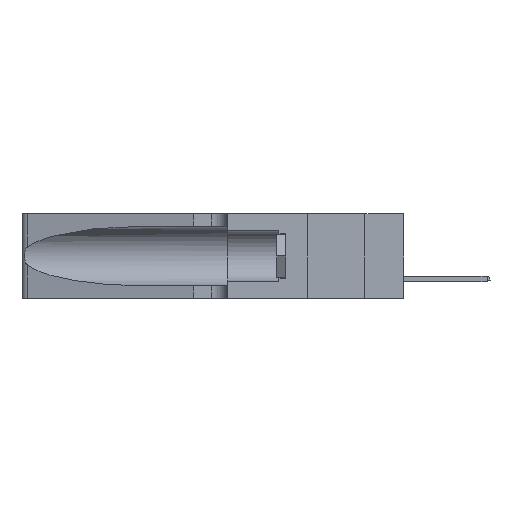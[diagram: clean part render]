
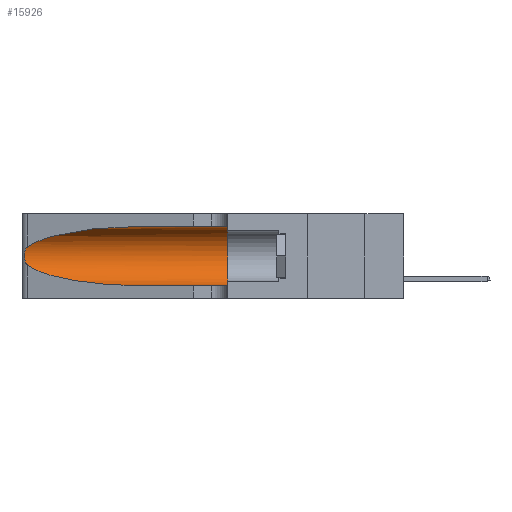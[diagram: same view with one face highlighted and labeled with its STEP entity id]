
A CAD part, left-side view. The second image highlights one B-rep face of the part: STEP entity #15926.
In plain terms, the highlighted cylindrical face has radius 3.308 mm (diameter 6.617 mm), a partial arc.
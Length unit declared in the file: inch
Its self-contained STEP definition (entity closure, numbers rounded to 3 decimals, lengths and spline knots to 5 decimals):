
#11 = ORIENTED_EDGE ( 'NONE', *, *, #22181, .T. ) ;
#1484 = LINE ( 'NONE', #30750, #23868 ) ;
#2147 = AXIS2_PLACEMENT_3D ( 'NONE', #30139, #44081, #11993 ) ;
#3268 = VECTOR ( 'NONE', #19122, 39.37008 ) ;
#3505 = CARTESIAN_POINT ( 'NONE',  ( 0.18966, 0.96281, 0.05475 ) ) ;
#4495 = VERTEX_POINT ( 'NONE', #6884 ) ;
#5133 = EDGE_CURVE ( 'NONE', #8652, #41421, #1484, .T. ) ;
#5287 = CARTESIAN_POINT ( 'NONE',  ( 0.1305, 0.72297, 0.31525 ) ) ;
#5605 = ORIENTED_EDGE ( 'NONE', *, *, #5133, .F. ) ;
#6344 = CARTESIAN_POINT ( 'NONE',  ( 0.25487, 1.22718, 0.22369 ) ) ;
#6884 = CARTESIAN_POINT ( 'NONE',  ( 0.1305, 0.35, 0.05475 ) ) ;
#8229 = CARTESIAN_POINT ( 'NONE',  ( 0.25639, 1.23184, 0.21858 ) ) ;
#8386 = CARTESIAN_POINT ( 'NONE',  ( 0.26018, 1.23835, 0.19895 ) ) ;
#8476 = CARTESIAN_POINT ( 'NONE',  ( 0.1305, 0.35, 0.31525 ) ) ;
#8652 = VERTEX_POINT ( 'NONE', #43155 ) ;
#11655 = CARTESIAN_POINT ( 'NONE',  ( 0.26017, 1.23833, 0.17102 ) ) ;
#11726 = VERTEX_POINT ( 'NONE', #19846 ) ;
#11993 = DIRECTION ( 'NONE',  ( 0., 0., 1. ) ) ;
#12289 = CARTESIAN_POINT ( 'NONE',  ( 0.25639, 1.23186, 0.15144 ) ) ;
#12607 = CARTESIAN_POINT ( 'NONE',  ( 0.2373, 1.15595, 0.28018 ) ) ;
#14136 = AXIS2_PLACEMENT_3D ( 'NONE', #37741, #41178, #19529 ) ;
#15405 = CARTESIAN_POINT ( 'NONE',  ( 0.26075, 1.23896, 0.19203 ) ) ;
#15566 = CARTESIAN_POINT ( 'NONE',  ( 0.25555, 1.22993, 0.14849 ) ) ;
#15838 = CYLINDRICAL_SURFACE ( 'NONE', #14136, 0.13025 ) ;
#15926 = ADVANCED_FACE ( 'NONE', ( #37762 ), #15838, .F. ) ;
#16428 = EDGE_CURVE ( 'NONE', #41421, #4495, #36569, .T. ) ;
#17183 = CARTESIAN_POINT ( 'NONE',  ( 0.1305, 0.72297, 0.05475 ) ) ;
#18900 = CARTESIAN_POINT ( 'NONE',  ( 0.25487, 1.22718, 0.14631 ) ) ;
#19122 = DIRECTION ( 'NONE',  ( 0., -1., 0. ) ) ;
#19529 = DIRECTION ( 'NONE',  ( 0., 0., -1. ) ) ;
#19846 = CARTESIAN_POINT ( 'NONE',  ( 0.25487, 1.22718, 0.14631 ) ) ;
#20450 = CARTESIAN_POINT ( 'NONE',  ( 0.25555, 1.22994, 0.2215 ) ) ;
#21374 = CARTESIAN_POINT ( 'NONE',  ( 0.1305, 0.72297, 0.05475 ) ) ;
#22181 = EDGE_CURVE ( 'NONE', #28431, #11726, #44897, .T. ) ;
#22808 = CARTESIAN_POINT ( 'NONE',  ( 0.2373, 1.15595, 0.08982 ) ) ;
#23224 = CARTESIAN_POINT ( 'NONE',  ( 0.25487, 1.22718, 0.22369 ) ) ;
#23688 = DIRECTION ( 'NONE',  ( 0., -1., 0. ) ) ;
#23868 = VECTOR ( 'NONE', #23688, 39.37008 ) ;
#24244 = EDGE_CURVE ( 'NONE', #32822, #4495, #30634, .T. ) ;
#26174 = CARTESIAN_POINT ( 'NONE',  ( 0.25487, 1.22718, 0.14631 ) ) ;
#26333 = CARTESIAN_POINT ( 'NONE',  ( 0.25789, 1.23486, 0.15765 ) ) ;
#26790 =( BOUNDED_CURVE ( )  B_SPLINE_CURVE ( 3, ( #5287, #37366, #12607, #23224 ),
 .UNSPECIFIED., .F., .T. ) 
 B_SPLINE_CURVE_WITH_KNOTS ( ( 4, 4 ),
 ( 1.5708, 2.84003 ),
 .UNSPECIFIED. ) 
 CURVE ( )  GEOMETRIC_REPRESENTATION_ITEM ( )  RATIONAL_B_SPLINE_CURVE ( ( 1., 0.87, 0.87, 1. ) ) 
 REPRESENTATION_ITEM ( '' )  );
#28431 = VERTEX_POINT ( 'NONE', #6344 ) ;
#29142 = CARTESIAN_POINT ( 'NONE',  ( 0.1305, 1.61858, 0.05475 ) ) ;
#30139 = CARTESIAN_POINT ( 'NONE',  ( 0.1305, 0.35, 0.185 ) ) ;
#30634 = LINE ( 'NONE', #29142, #3268 ) ;
#30750 = CARTESIAN_POINT ( 'NONE',  ( 0.1305, 1.61858, 0.31525 ) ) ;
#32822 = VERTEX_POINT ( 'NONE', #17183 ) ;
#33107 = CARTESIAN_POINT ( 'NONE',  ( 0.25787, 1.23484, 0.2124 ) ) ;
#34504 = ORIENTED_EDGE ( 'NONE', *, *, #16428, .F. ) ;
#36569 = CIRCLE ( 'NONE', #2147, 0.13025 ) ;
#36736 = CARTESIAN_POINT ( 'NONE',  ( 0.26075, 1.23896, 0.178 ) ) ;
#37052 = CARTESIAN_POINT ( 'NONE',  ( 0.25856, 1.23593, 0.16098 ) ) ;
#37366 = CARTESIAN_POINT ( 'NONE',  ( 0.18966, 0.96281, 0.31525 ) ) ;
#37697 = EDGE_CURVE ( 'NONE', #8652, #28431, #26790, .T. ) ;
#37741 = CARTESIAN_POINT ( 'NONE',  ( 0.1305, 1.61858, 0.185 ) ) ;
#37762 = FACE_OUTER_BOUND ( 'NONE', #42913, .T. ) ;
#40598 = EDGE_CURVE ( 'NONE', #11726, #32822, #42646, .T. ) ;
#40662 = CARTESIAN_POINT ( 'NONE',  ( 0.25854, 1.2359, 0.20912 ) ) ;
#40750 = ORIENTED_EDGE ( 'NONE', *, *, #40598, .T. ) ;
#40962 = ORIENTED_EDGE ( 'NONE', *, *, #37697, .T. ) ;
#41116 = ORIENTED_EDGE ( 'NONE', *, *, #24244, .T. ) ;
#41178 = DIRECTION ( 'NONE',  ( 0., -1., 0. ) ) ;
#41421 = VERTEX_POINT ( 'NONE', #8476 ) ;
#42646 =( BOUNDED_CURVE ( )  B_SPLINE_CURVE ( 3, ( #18900, #22808, #3505, #21374 ),
 .UNSPECIFIED., .F., .F. ) 
 B_SPLINE_CURVE_WITH_KNOTS ( ( 4, 4 ),
 ( 3.44316, 4.71239 ),
 .UNSPECIFIED. ) 
 CURVE ( )  GEOMETRIC_REPRESENTATION_ITEM ( )  RATIONAL_B_SPLINE_CURVE ( ( 1., 0.87, 0.87, 1. ) ) 
 REPRESENTATION_ITEM ( '' )  );
#42913 = EDGE_LOOP ( 'NONE', ( #40962, #11, #40750, #41116, #34504, #5605 ) ) ;
#43155 = CARTESIAN_POINT ( 'NONE',  ( 0.1305, 0.72297, 0.31525 ) ) ;
#44081 = DIRECTION ( 'NONE',  ( 0., 1., 0. ) ) ;
#44897 = B_SPLINE_CURVE_WITH_KNOTS ( 'NONE', 3,
 ( #46260, #20450, #8229, #33107, #40662, #8386, #15405, #36736, #11655, #37052, #26333, #12289, #15566, #26174 ),
 .UNSPECIFIED., .F., .F.,
 ( 4, 2, 2, 2, 2, 2, 4 ),
 ( 0., 0.00027, 0.00053, 0.00107, 0.0016, 0.00187, 0.00214 ),
 .UNSPECIFIED. ) ;
#46260 = CARTESIAN_POINT ( 'NONE',  ( 0.25487, 1.22718, 0.22369 ) ) ;
